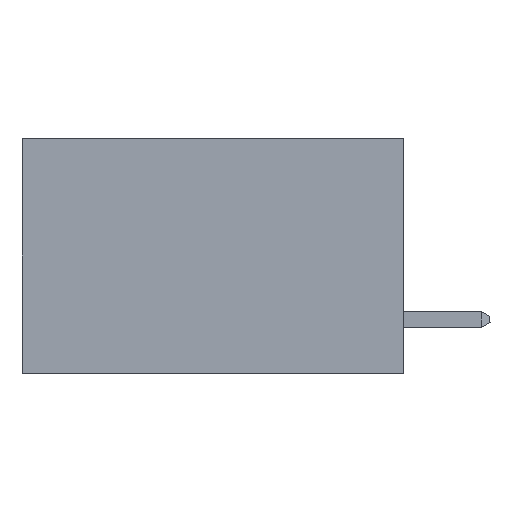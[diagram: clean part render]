
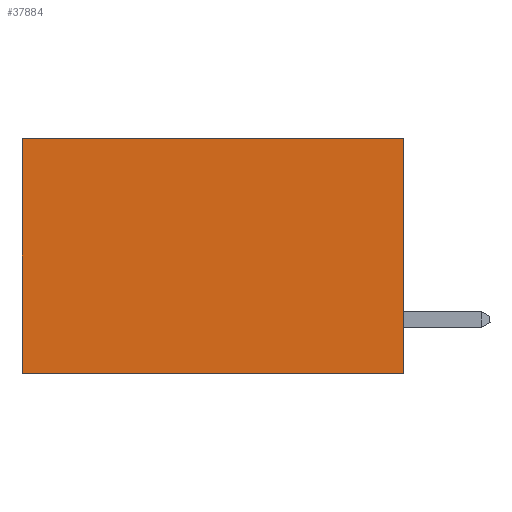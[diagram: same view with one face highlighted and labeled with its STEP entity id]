
A CAD part, left-side view. The second image highlights one B-rep face of the part: STEP entity #37884.
In plain terms, the highlighted planar face has unit normal (-1, 0, 0).
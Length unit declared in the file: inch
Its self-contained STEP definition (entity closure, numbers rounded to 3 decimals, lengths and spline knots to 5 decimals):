
#165 = AXIS2_PLACEMENT_3D ( 'NONE', #37525, #18493, #40632 ) ;
#1949 = EDGE_CURVE ( 'NONE', #36927, #41196, #28926, .T. ) ;
#2783 = CARTESIAN_POINT ( 'NONE',  ( 0.2875, 0.6, -0.37 ) ) ;
#2793 = LINE ( 'NONE', #13444, #18924 ) ;
#3240 = ORIENTED_EDGE ( 'NONE', *, *, #1949, .F. ) ;
#3247 = VECTOR ( 'NONE', #9076, 39.37008 ) ;
#3372 = ORIENTED_EDGE ( 'NONE', *, *, #32785, .F. ) ;
#4566 = EDGE_LOOP ( 'NONE', ( #31826, #3372, #3240, #31806 ) ) ;
#6493 = VECTOR ( 'NONE', #32405, 39.37008 ) ;
#8153 = CARTESIAN_POINT ( 'NONE',  ( 0.2875, 0., -0.37 ) ) ;
#8814 = CARTESIAN_POINT ( 'NONE',  ( 0.2875, 0., 0. ) ) ;
#9076 = DIRECTION ( 'NONE',  ( 0., 0., -1. ) ) ;
#10239 = CARTESIAN_POINT ( 'NONE',  ( 0.2875, 0., 0. ) ) ;
#12471 = VERTEX_POINT ( 'NONE', #2783 ) ;
#13015 = CARTESIAN_POINT ( 'NONE',  ( 0.2875, 0., -0.37 ) ) ;
#13444 = CARTESIAN_POINT ( 'NONE',  ( 0.2875, 0., 0. ) ) ;
#13952 = CARTESIAN_POINT ( 'NONE',  ( 0.2875, 0.6, 0. ) ) ;
#17306 = DIRECTION ( 'NONE',  ( 0., 0., -1. ) ) ;
#18493 = DIRECTION ( 'NONE',  ( 1., 0., 0. ) ) ;
#18924 = VECTOR ( 'NONE', #32808, 39.37008 ) ;
#21600 = LINE ( 'NONE', #13952, #37390 ) ;
#25499 = CARTESIAN_POINT ( 'NONE',  ( 0.2875, 0.6, 0. ) ) ;
#28045 = PLANE ( 'NONE',  #165 ) ;
#28794 = FACE_OUTER_BOUND ( 'NONE', #4566, .T. ) ;
#28926 = LINE ( 'NONE', #8814, #3247 ) ;
#31806 = ORIENTED_EDGE ( 'NONE', *, *, #36251, .T. ) ;
#31826 = ORIENTED_EDGE ( 'NONE', *, *, #35125, .T. ) ;
#32180 = LINE ( 'NONE', #13015, #6493 ) ;
#32405 = DIRECTION ( 'NONE',  ( 0., 1., 0. ) ) ;
#32785 = EDGE_CURVE ( 'NONE', #41196, #12471, #32180, .T. ) ;
#32808 = DIRECTION ( 'NONE',  ( 0., 1., 0. ) ) ;
#35125 = EDGE_CURVE ( 'NONE', #40810, #12471, #21600, .T. ) ;
#36251 = EDGE_CURVE ( 'NONE', #36927, #40810, #2793, .T. ) ;
#36927 = VERTEX_POINT ( 'NONE', #10239 ) ;
#37390 = VECTOR ( 'NONE', #17306, 39.37008 ) ;
#37525 = CARTESIAN_POINT ( 'NONE',  ( 0.2875, 0., 0. ) ) ;
#37884 = ADVANCED_FACE ( 'NONE', ( #28794 ), #28045, .F. ) ;
#40632 = DIRECTION ( 'NONE',  ( 0., 0., -1. ) ) ;
#40810 = VERTEX_POINT ( 'NONE', #25499 ) ;
#41196 = VERTEX_POINT ( 'NONE', #8153 ) ;
